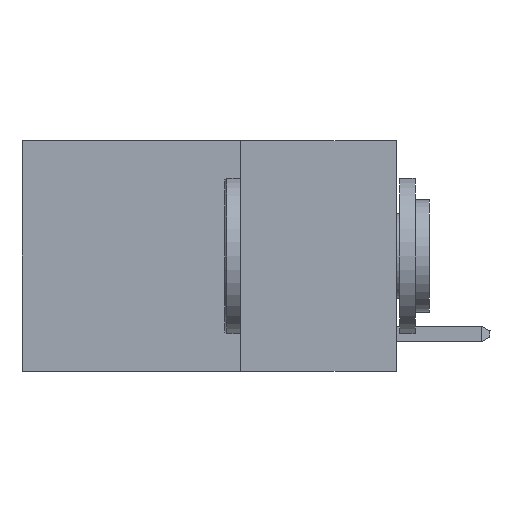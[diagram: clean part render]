
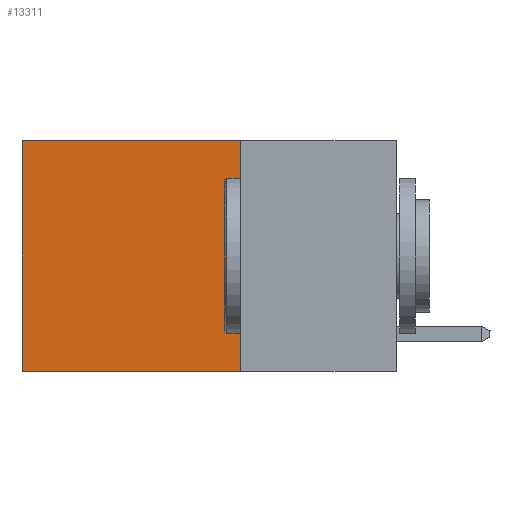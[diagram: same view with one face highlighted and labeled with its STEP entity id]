
A CAD part, left-side view. The second image highlights one B-rep face of the part: STEP entity #13311.
In plain terms, the highlighted planar face has unit normal (-1, 0, 0).
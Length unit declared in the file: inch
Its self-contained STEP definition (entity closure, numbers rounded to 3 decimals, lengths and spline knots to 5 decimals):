
#271 = PLANE ( 'NONE',  #11080 ) ;
#456 = VERTEX_POINT ( 'NONE', #14014 ) ;
#981 = DIRECTION ( 'NONE',  ( 0., 1., 0. ) ) ;
#1330 = VECTOR ( 'NONE', #18137, 39.37008 ) ;
#1513 = VERTEX_POINT ( 'NONE', #2863 ) ;
#2776 = LINE ( 'NONE', #10531, #1330 ) ;
#2863 = CARTESIAN_POINT ( 'NONE',  ( 0.2625, 0.6, 0. ) ) ;
#3047 = EDGE_CURVE ( 'NONE', #9320, #7990, #2776, .T. ) ;
#3218 = LINE ( 'NONE', #15737, #14295 ) ;
#3278 = EDGE_CURVE ( 'NONE', #7990, #456, #14782, .T. ) ;
#3689 = ORIENTED_EDGE ( 'NONE', *, *, #3278, .F. ) ;
#4699 = DIRECTION ( 'NONE',  ( 0., 0., -1. ) ) ;
#5577 = EDGE_CURVE ( 'NONE', #9320, #1513, #17052, .T. ) ;
#6307 = DIRECTION ( 'NONE',  ( 0., 1., 0. ) ) ;
#6469 = DIRECTION ( 'NONE',  ( 0., 0., -1. ) ) ;
#6477 = ORIENTED_EDGE ( 'NONE', *, *, #5577, .T. ) ;
#6541 = VECTOR ( 'NONE', #981, 39.37008 ) ;
#7990 = VERTEX_POINT ( 'NONE', #16436 ) ;
#8060 = CARTESIAN_POINT ( 'NONE',  ( 0.2625, 0.25, 0. ) ) ;
#9320 = VERTEX_POINT ( 'NONE', #11950 ) ;
#10531 = CARTESIAN_POINT ( 'NONE',  ( 0.2625, 0.25, 0. ) ) ;
#10985 = CARTESIAN_POINT ( 'NONE',  ( 0.2625, 0.25, 0. ) ) ;
#11080 = AXIS2_PLACEMENT_3D ( 'NONE', #10985, #12421, #4699 ) ;
#11766 = VECTOR ( 'NONE', #6307, 39.37008 ) ;
#11950 = CARTESIAN_POINT ( 'NONE',  ( 0.2625, 0.25, 0. ) ) ;
#12421 = DIRECTION ( 'NONE',  ( 1., 0., 0. ) ) ;
#13311 = ADVANCED_FACE ( 'NONE', ( #18352 ), #271, .F. ) ;
#13740 = EDGE_LOOP ( 'NONE', ( #14162, #3689, #14687, #6477 ) ) ;
#14014 = CARTESIAN_POINT ( 'NONE',  ( 0.2625, 0.6, -0.37 ) ) ;
#14162 = ORIENTED_EDGE ( 'NONE', *, *, #15806, .T. ) ;
#14295 = VECTOR ( 'NONE', #6469, 39.37008 ) ;
#14687 = ORIENTED_EDGE ( 'NONE', *, *, #3047, .F. ) ;
#14782 = LINE ( 'NONE', #19412, #6541 ) ;
#15737 = CARTESIAN_POINT ( 'NONE',  ( 0.2625, 0.6, 0. ) ) ;
#15806 = EDGE_CURVE ( 'NONE', #1513, #456, #3218, .T. ) ;
#16436 = CARTESIAN_POINT ( 'NONE',  ( 0.2625, 0.25, -0.37 ) ) ;
#17052 = LINE ( 'NONE', #8060, #11766 ) ;
#18137 = DIRECTION ( 'NONE',  ( 0., 0., -1. ) ) ;
#18352 = FACE_OUTER_BOUND ( 'NONE', #13740, .T. ) ;
#19412 = CARTESIAN_POINT ( 'NONE',  ( 0.2625, 0.25, -0.37 ) ) ;
